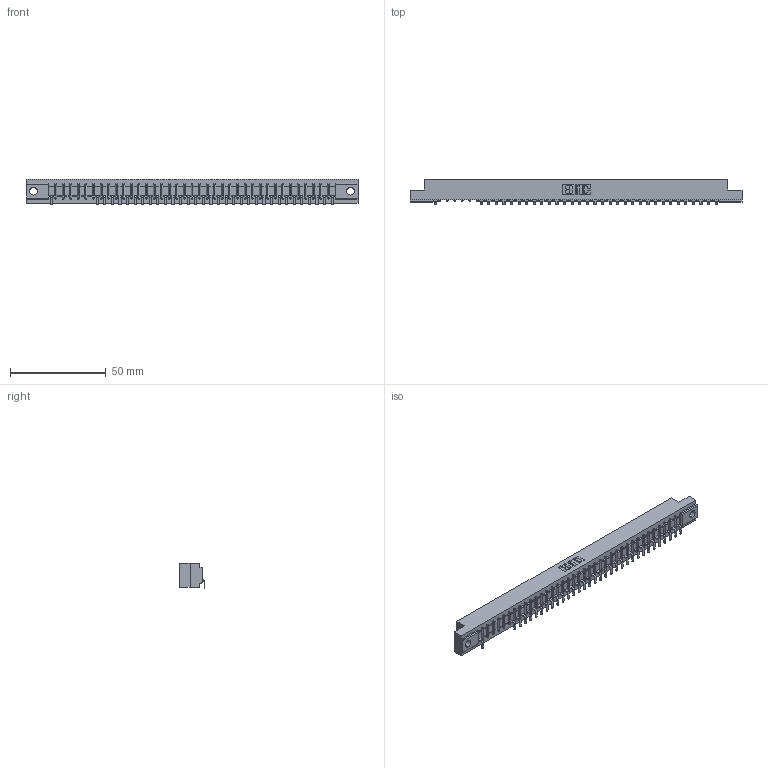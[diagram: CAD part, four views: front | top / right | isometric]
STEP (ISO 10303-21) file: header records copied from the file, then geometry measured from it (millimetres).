
FILE_DESCRIPTION (( 'STEP AP203' ), '1' );
FILE_NAME ('357-038-553-104.STEP', '2018-08-10T09:21:09', ( '' ), ( '' ), 'SwSTEP 2.0', 'SolidWorks 2016', '' );
FILE_SCHEMA (( 'CONFIG_CONTROL_DESIGN' ));
Length unit declared in the file: inch
Products named in the file (3): 307 Part_.156 Dia Mounting Holes; 307-290-002_553; 357-038-553-104
Assembly tree (34 placements, depth 2):
  357-038-553-104
    307 Part_.156 Dia Mounting Holes
    307-290-002_553  x33
Bounding box: 173.58 x 13.32 x 13.5 mm (x, y, z)
Volume: 18295 mm3; surface area: 21819.4 mm2
Topology: 34 solids, 34 shells, 2845 faces, 8731 edges, 5714 vertices
Faces by surface type: plane 1695, cylinder 1072, sphere 78
Entity records: 34182 total; most frequent: CARTESIAN_POINT 5793, ORIENTED_EDGE 5786, DIRECTION 5617, EDGE_CURVE 2893, VECTOR 2221, LINE 2221, VERTEX_POINT 1874, AXIS2_PLACEMENT_3D 1698
